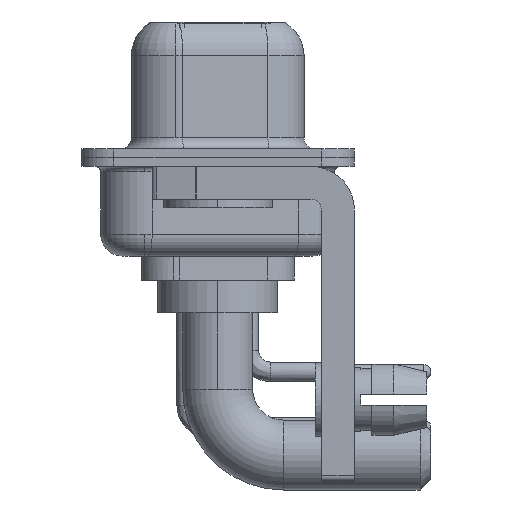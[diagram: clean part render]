
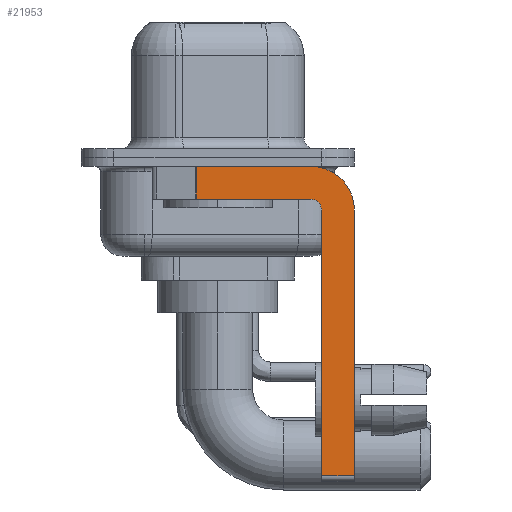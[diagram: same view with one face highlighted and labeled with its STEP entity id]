
A CAD part, left-side view. The second image highlights one B-rep face of the part: STEP entity #21953.
In plain terms, the highlighted planar face has unit normal (-1, 0, 0).
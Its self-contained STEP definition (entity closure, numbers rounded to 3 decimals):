
#456 = EDGE_CURVE ( 'NONE', #11078, #6788, #14515, .T. ) ;
#605 = EDGE_LOOP ( 'NONE', ( #8153, #4751, #21934, #19185, #23528, #1252, #5410, #2202 ) ) ;
#1252 = ORIENTED_EDGE ( 'NONE', *, *, #18344, .T. ) ;
#2071 = DIRECTION ( 'NONE',  ( 0., -1., 0. ) ) ;
#2202 = ORIENTED_EDGE ( 'NONE', *, *, #12123, .F. ) ;
#2418 = CARTESIAN_POINT ( 'NONE',  ( -2.9, -6.25, -2.4 ) ) ;
#2596 = DIRECTION ( 'NONE',  ( 0., 0., 1. ) ) ;
#3093 = CARTESIAN_POINT ( 'NONE',  ( -2.9, -6.25, -14.55 ) ) ;
#3421 = VECTOR ( 'NONE', #2071, 1000. ) ;
#3446 = VERTEX_POINT ( 'NONE', #25242 ) ;
#3538 = VECTOR ( 'NONE', #5187, 1000. ) ;
#4066 = CIRCLE ( 'NONE', #6692, 0.5 ) ;
#4193 = CARTESIAN_POINT ( 'NONE',  ( -2.9, -4.75, -2.4 ) ) ;
#4212 = DIRECTION ( 'NONE',  ( 0., 0., -1. ) ) ;
#4326 = DIRECTION ( 'NONE',  ( 0., 0., -1. ) ) ;
#4616 = VECTOR ( 'NONE', #20942, 1000. ) ;
#4751 = ORIENTED_EDGE ( 'NONE', *, *, #6374, .T. ) ;
#5187 = DIRECTION ( 'NONE',  ( 0., 0., -1. ) ) ;
#5202 = VERTEX_POINT ( 'NONE', #4193 ) ;
#5410 = ORIENTED_EDGE ( 'NONE', *, *, #456, .F. ) ;
#5877 = CARTESIAN_POINT ( 'NONE',  ( -2.9, -6.25, -2.4 ) ) ;
#6198 = LINE ( 'NONE', #14569, #3421 ) ;
#6374 = EDGE_CURVE ( 'NONE', #11595, #13160, #26111, .T. ) ;
#6692 = AXIS2_PLACEMENT_3D ( 'NONE', #16608, #14424, #18823 ) ;
#6788 = VERTEX_POINT ( 'NONE', #3093 ) ;
#6927 = VECTOR ( 'NONE', #2596, 1000. ) ;
#7420 = CARTESIAN_POINT ( 'NONE',  ( -2.9, -4.25, -2.4 ) ) ;
#7449 = CARTESIAN_POINT ( 'NONE',  ( -2.9, -4.25, -1.9 ) ) ;
#8153 = ORIENTED_EDGE ( 'NONE', *, *, #15261, .F. ) ;
#8666 = CIRCLE ( 'NONE', #24034, 2. ) ;
#11078 = VERTEX_POINT ( 'NONE', #2418 ) ;
#11595 = VERTEX_POINT ( 'NONE', #25488 ) ;
#12123 = EDGE_CURVE ( 'NONE', #21237, #11078, #8666, .T. ) ;
#13043 = CARTESIAN_POINT ( 'NONE',  ( -2.9, -4.75, -14.8 ) ) ;
#13160 = VERTEX_POINT ( 'NONE', #27124 ) ;
#14424 = DIRECTION ( 'NONE',  ( -1., 0., 0. ) ) ;
#14515 = LINE ( 'NONE', #5877, #25883 ) ;
#14569 = CARTESIAN_POINT ( 'NONE',  ( -2.9, -4.25, -14.55 ) ) ;
#14697 = VERTEX_POINT ( 'NONE', #7449 ) ;
#14892 = EDGE_CURVE ( 'NONE', #14697, #13160, #23279, .T. ) ;
#15094 = LINE ( 'NONE', #13043, #6927 ) ;
#15261 = EDGE_CURVE ( 'NONE', #11595, #21237, #16899, .T. ) ;
#15718 = CARTESIAN_POINT ( 'NONE',  ( -2.9, -4.25, -0.4 ) ) ;
#15794 = DIRECTION ( 'NONE',  ( 1., 0., 0. ) ) ;
#16608 = CARTESIAN_POINT ( 'NONE',  ( -2.9, -4.25, -2.4 ) ) ;
#16899 = LINE ( 'NONE', #18712, #17814 ) ;
#17375 = EDGE_CURVE ( 'NONE', #3446, #5202, #15094, .T. ) ;
#17619 = AXIS2_PLACEMENT_3D ( 'NONE', #20590, #23057, #4212 ) ;
#17693 = CARTESIAN_POINT ( 'NONE',  ( -2.9, 0.978, -1.9 ) ) ;
#17814 = VECTOR ( 'NONE', #20787, 1000. ) ;
#18344 = EDGE_CURVE ( 'NONE', #3446, #6788, #6198, .T. ) ;
#18712 = CARTESIAN_POINT ( 'NONE',  ( -2.9, 3., -0.4 ) ) ;
#18742 = CARTESIAN_POINT ( 'NONE',  ( -2.9, -4.25, -1.9 ) ) ;
#18823 = DIRECTION ( 'NONE',  ( 0., 0., 1. ) ) ;
#19185 = ORIENTED_EDGE ( 'NONE', *, *, #22771, .F. ) ;
#20590 = CARTESIAN_POINT ( 'NONE',  ( -2.9, -4.25, -2.4 ) ) ;
#20787 = DIRECTION ( 'NONE',  ( 0., -1., 0. ) ) ;
#20942 = DIRECTION ( 'NONE',  ( 0., 1., 0. ) ) ;
#21237 = VERTEX_POINT ( 'NONE', #15718 ) ;
#21934 = ORIENTED_EDGE ( 'NONE', *, *, #14892, .F. ) ;
#21953 = ADVANCED_FACE ( 'NONE', ( #22661 ), #25137, .F. ) ;
#22661 = FACE_OUTER_BOUND ( 'NONE', #605, .T. ) ;
#22771 = EDGE_CURVE ( 'NONE', #5202, #14697, #4066, .T. ) ;
#23057 = DIRECTION ( 'NONE',  ( 1., 0., 0. ) ) ;
#23279 = LINE ( 'NONE', #18742, #4616 ) ;
#23528 = ORIENTED_EDGE ( 'NONE', *, *, #17375, .F. ) ;
#24034 = AXIS2_PLACEMENT_3D ( 'NONE', #7420, #15794, #24335 ) ;
#24335 = DIRECTION ( 'NONE',  ( 0., 0., -1. ) ) ;
#25137 = PLANE ( 'NONE',  #17619 ) ;
#25242 = CARTESIAN_POINT ( 'NONE',  ( -2.9, -4.75, -14.55 ) ) ;
#25488 = CARTESIAN_POINT ( 'NONE',  ( -2.9, 0.978, -0.4 ) ) ;
#25883 = VECTOR ( 'NONE', #4326, 1000. ) ;
#26111 = LINE ( 'NONE', #17693, #3538 ) ;
#27124 = CARTESIAN_POINT ( 'NONE',  ( -2.9, 0.978, -1.9 ) ) ;
